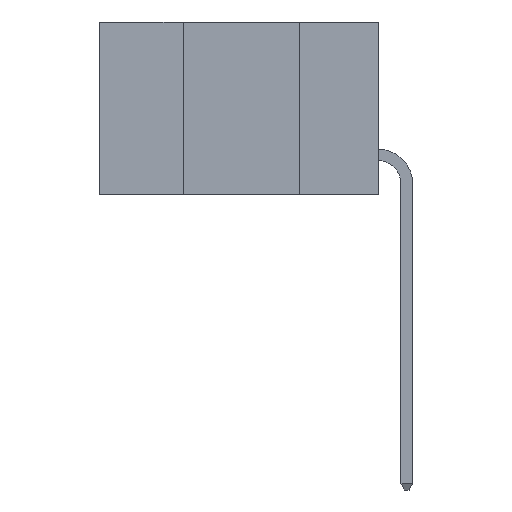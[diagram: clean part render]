
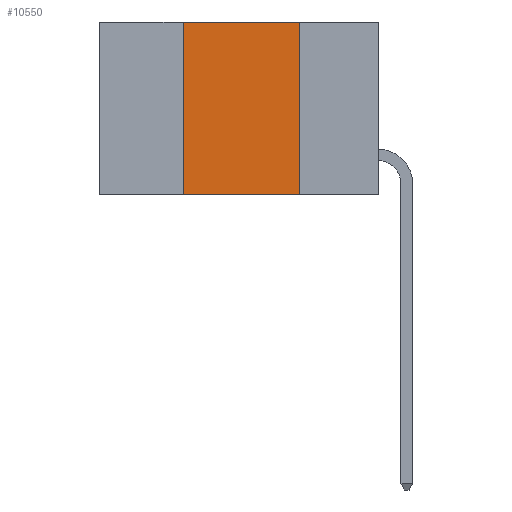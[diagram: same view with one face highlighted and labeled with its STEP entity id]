
A CAD part, left-side view. The second image highlights one B-rep face of the part: STEP entity #10550.
In plain terms, the highlighted planar face has unit normal (-1, 0, 0).
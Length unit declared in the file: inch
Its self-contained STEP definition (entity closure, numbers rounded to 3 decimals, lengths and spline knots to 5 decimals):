
#30 = CARTESIAN_POINT ( 'NONE',  ( 0., 0.6, 0. ) ) ;
#1375 = DIRECTION ( 'NONE',  ( 1., 0., 0. ) ) ;
#2780 = EDGE_CURVE ( 'NONE', #12714, #7208, #16317, .T. ) ;
#2874 = VECTOR ( 'NONE', #4251, 39.37008 ) ;
#3104 = EDGE_CURVE ( 'NONE', #6417, #12714, #4867, .T. ) ;
#3240 = ORIENTED_EDGE ( 'NONE', *, *, #13514, .F. ) ;
#3605 = ORIENTED_EDGE ( 'NONE', *, *, #2780, .F. ) ;
#3696 = ORIENTED_EDGE ( 'NONE', *, *, #3104, .F. ) ;
#3920 = ORIENTED_EDGE ( 'NONE', *, *, #7222, .T. ) ;
#4251 = DIRECTION ( 'NONE',  ( 0., -1., 0. ) ) ;
#4344 = VECTOR ( 'NONE', #6776, 39.37008 ) ;
#4433 = CARTESIAN_POINT ( 'NONE',  ( 0., 0.42, 0. ) ) ;
#4867 = LINE ( 'NONE', #15436, #14550 ) ;
#5034 = AXIS2_PLACEMENT_3D ( 'NONE', #30, #1375, #10305 ) ;
#5141 = CARTESIAN_POINT ( 'NONE',  ( 0., 0.6, 0. ) ) ;
#5713 = FACE_OUTER_BOUND ( 'NONE', #9429, .T. ) ;
#6080 = DIRECTION ( 'NONE',  ( 0., 0., -1. ) ) ;
#6417 = VERTEX_POINT ( 'NONE', #13790 ) ;
#6717 = CARTESIAN_POINT ( 'NONE',  ( 0., 0.17, 0. ) ) ;
#6776 = DIRECTION ( 'NONE',  ( 0., -1., 0. ) ) ;
#6838 = VERTEX_POINT ( 'NONE', #12363 ) ;
#7208 = VERTEX_POINT ( 'NONE', #6717 ) ;
#7222 = EDGE_CURVE ( 'NONE', #6417, #6838, #11076, .T. ) ;
#9429 = EDGE_LOOP ( 'NONE', ( #3240, #3605, #3696, #3920 ) ) ;
#10305 = DIRECTION ( 'NONE',  ( 0., 0., -1. ) ) ;
#10550 = ADVANCED_FACE ( 'NONE', ( #5713 ), #15315, .F. ) ;
#11076 = LINE ( 'NONE', #13063, #4344 ) ;
#11730 = VECTOR ( 'NONE', #6080, 39.37008 ) ;
#12363 = CARTESIAN_POINT ( 'NONE',  ( 0., 0.17, -0.37 ) ) ;
#12714 = VERTEX_POINT ( 'NONE', #4433 ) ;
#13063 = CARTESIAN_POINT ( 'NONE',  ( 0., 0.6, -0.37 ) ) ;
#13514 = EDGE_CURVE ( 'NONE', #7208, #6838, #15071, .T. ) ;
#13790 = CARTESIAN_POINT ( 'NONE',  ( 0., 0.42, -0.37 ) ) ;
#14550 = VECTOR ( 'NONE', #15525, 39.37008 ) ;
#15071 = LINE ( 'NONE', #16098, #11730 ) ;
#15315 = PLANE ( 'NONE',  #5034 ) ;
#15436 = CARTESIAN_POINT ( 'NONE',  ( 0., 0.42, -0.37 ) ) ;
#15525 = DIRECTION ( 'NONE',  ( 0., 0., 1. ) ) ;
#16098 = CARTESIAN_POINT ( 'NONE',  ( 0., 0.17, -0.37 ) ) ;
#16317 = LINE ( 'NONE', #5141, #2874 ) ;
